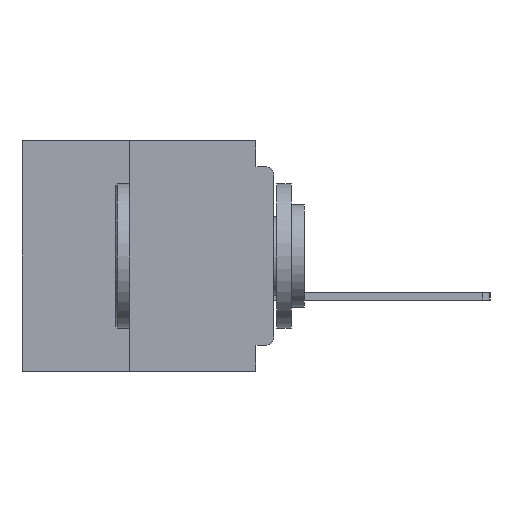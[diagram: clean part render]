
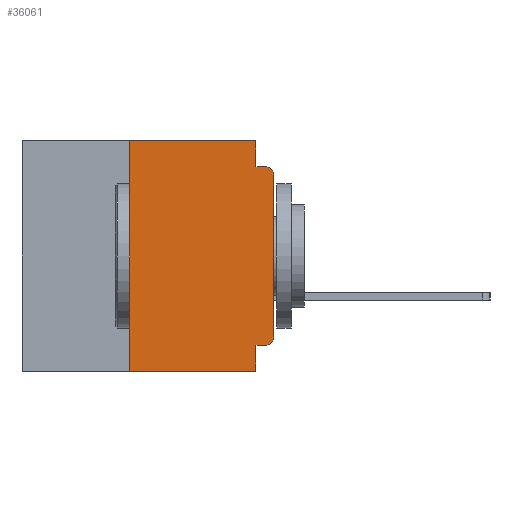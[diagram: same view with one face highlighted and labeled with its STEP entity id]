
A CAD part, left-side view. The second image highlights one B-rep face of the part: STEP entity #36061.
In plain terms, the highlighted planar face has unit normal (-1, 0, 0).
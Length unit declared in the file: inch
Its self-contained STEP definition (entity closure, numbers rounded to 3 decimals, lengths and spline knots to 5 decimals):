
#31 = DIRECTION ( 'NONE',  ( 0., -1., 0. ) ) ;
#459 = ORIENTED_EDGE ( 'NONE', *, *, #33806, .T. ) ;
#517 = DIRECTION ( 'NONE',  ( 0., 0., -1. ) ) ;
#1247 = DIRECTION ( 'NONE',  ( 0., -1., 0. ) ) ;
#2283 = LINE ( 'NONE', #17625, #20515 ) ;
#2712 = VERTEX_POINT ( 'NONE', #13226 ) ;
#4377 = CARTESIAN_POINT ( 'NONE',  ( 0., 0.031, -0.045 ) ) ;
#5106 = VERTEX_POINT ( 'NONE', #21611 ) ;
#5412 = ORIENTED_EDGE ( 'NONE', *, *, #19987, .T. ) ;
#6011 = AXIS2_PLACEMENT_3D ( 'NONE', #10459, #39322, #14601 ) ;
#7656 = CARTESIAN_POINT ( 'NONE',  ( 0., 0.031, 0. ) ) ;
#8273 = LINE ( 'NONE', #52745, #50850 ) ;
#10038 = DIRECTION ( 'NONE',  ( -1., 0., 0. ) ) ;
#10459 = CARTESIAN_POINT ( 'NONE',  ( 0., 0.015, -0.34 ) ) ;
#11101 = VERTEX_POINT ( 'NONE', #41931 ) ;
#11694 = DIRECTION ( 'NONE',  ( 0., 1., 0. ) ) ;
#13226 = CARTESIAN_POINT ( 'NONE',  ( 0., 0., -0.06 ) ) ;
#13695 = CARTESIAN_POINT ( 'NONE',  ( 0., 0.437, 0. ) ) ;
#14601 = DIRECTION ( 'NONE',  ( 0., 0., -1. ) ) ;
#14728 = LINE ( 'NONE', #50128, #35390 ) ;
#15181 = VERTEX_POINT ( 'NONE', #52585 ) ;
#15403 = VERTEX_POINT ( 'NONE', #4377 ) ;
#15664 = DIRECTION ( 'NONE',  ( 0., -1., 0. ) ) ;
#15763 = CIRCLE ( 'NONE', #19614, 0.015 ) ;
#16553 = CARTESIAN_POINT ( 'NONE',  ( 0., 0.437, 0. ) ) ;
#16823 = EDGE_LOOP ( 'NONE', ( #44016, #459, #50328, #39913, #51917, #40638, #39721, #34998, #29249, #5412 ) ) ;
#17018 = CARTESIAN_POINT ( 'NONE',  ( 0., 0.015, -0.045 ) ) ;
#17625 = CARTESIAN_POINT ( 'NONE',  ( 0., 0.25, -0.4 ) ) ;
#18974 = EDGE_CURVE ( 'NONE', #15403, #24343, #45887, .T. ) ;
#19614 = AXIS2_PLACEMENT_3D ( 'NONE', #34772, #10038, #38875 ) ;
#19987 = EDGE_CURVE ( 'NONE', #5106, #11101, #48443, .T. ) ;
#20515 = VECTOR ( 'NONE', #21734, 39.37008 ) ;
#20682 = DIRECTION ( 'NONE',  ( 0., 0., -1. ) ) ;
#21370 = CARTESIAN_POINT ( 'NONE',  ( 0., 0., 0. ) ) ;
#21611 = CARTESIAN_POINT ( 'NONE',  ( 0., 0.015, -0.355 ) ) ;
#21734 = DIRECTION ( 'NONE',  ( 0., 0., 1. ) ) ;
#22354 = EDGE_CURVE ( 'NONE', #48712, #46539, #46209, .T. ) ;
#22435 = AXIS2_PLACEMENT_3D ( 'NONE', #16553, #45345, #20682 ) ;
#22874 = VECTOR ( 'NONE', #15664, 39.37008 ) ;
#24320 = VECTOR ( 'NONE', #11694, 39.37008 ) ;
#24343 = VERTEX_POINT ( 'NONE', #17018 ) ;
#24941 = CARTESIAN_POINT ( 'NONE',  ( 0., 0., -0.045 ) ) ;
#24942 = CARTESIAN_POINT ( 'NONE',  ( 0., 0.25, -0.4 ) ) ;
#25096 = LINE ( 'NONE', #21370, #34847 ) ;
#25546 = VERTEX_POINT ( 'NONE', #24942 ) ;
#27867 = VECTOR ( 'NONE', #31, 39.37008 ) ;
#29249 = ORIENTED_EDGE ( 'NONE', *, *, #50360, .F. ) ;
#30649 = EDGE_CURVE ( 'NONE', #15181, #52900, #8273, .T. ) ;
#33409 = EDGE_CURVE ( 'NONE', #25546, #52900, #33882, .T. ) ;
#33686 = CARTESIAN_POINT ( 'NONE',  ( 0., 0.25, 0. ) ) ;
#33806 = EDGE_CURVE ( 'NONE', #2712, #24343, #15763, .T. ) ;
#33882 = LINE ( 'NONE', #36231, #22874 ) ;
#34772 = CARTESIAN_POINT ( 'NONE',  ( 0., 0.015, -0.06 ) ) ;
#34847 = VECTOR ( 'NONE', #46019, 39.37008 ) ;
#34998 = ORIENTED_EDGE ( 'NONE', *, *, #30649, .F. ) ;
#35305 = VECTOR ( 'NONE', #1247, 39.37008 ) ;
#35390 = VECTOR ( 'NONE', #517, 39.37008 ) ;
#36061 = ADVANCED_FACE ( 'NONE', ( #43195 ), #37090, .F. ) ;
#36231 = CARTESIAN_POINT ( 'NONE',  ( 0., 0.437, -0.4 ) ) ;
#36389 = DIRECTION ( 'NONE',  ( 0., 0., -1. ) ) ;
#37090 = PLANE ( 'NONE',  #22435 ) ;
#37526 = CARTESIAN_POINT ( 'NONE',  ( 0., 0.031, -0.4 ) ) ;
#38875 = DIRECTION ( 'NONE',  ( 0., 0., -1. ) ) ;
#39322 = DIRECTION ( 'NONE',  ( -1., 0., 0. ) ) ;
#39721 = ORIENTED_EDGE ( 'NONE', *, *, #33409, .T. ) ;
#39913 = ORIENTED_EDGE ( 'NONE', *, *, #49967, .F. ) ;
#40638 = ORIENTED_EDGE ( 'NONE', *, *, #44411, .F. ) ;
#41931 = CARTESIAN_POINT ( 'NONE',  ( 0., 0., -0.34 ) ) ;
#43195 = FACE_OUTER_BOUND ( 'NONE', #16823, .T. ) ;
#44016 = ORIENTED_EDGE ( 'NONE', *, *, #49343, .T. ) ;
#44411 = EDGE_CURVE ( 'NONE', #25546, #48712, #2283, .T. ) ;
#45345 = DIRECTION ( 'NONE',  ( 1., 0., 0. ) ) ;
#45887 = LINE ( 'NONE', #24941, #27867 ) ;
#46019 = DIRECTION ( 'NONE',  ( 0., 0., 1. ) ) ;
#46209 = LINE ( 'NONE', #13695, #35305 ) ;
#46539 = VERTEX_POINT ( 'NONE', #7656 ) ;
#47573 = LINE ( 'NONE', #52794, #24320 ) ;
#48443 = CIRCLE ( 'NONE', #6011, 0.015 ) ;
#48712 = VERTEX_POINT ( 'NONE', #33686 ) ;
#49343 = EDGE_CURVE ( 'NONE', #11101, #2712, #25096, .T. ) ;
#49967 = EDGE_CURVE ( 'NONE', #46539, #15403, #14728, .T. ) ;
#50128 = CARTESIAN_POINT ( 'NONE',  ( 0., 0.031, 0. ) ) ;
#50328 = ORIENTED_EDGE ( 'NONE', *, *, #18974, .F. ) ;
#50360 = EDGE_CURVE ( 'NONE', #5106, #15181, #47573, .T. ) ;
#50850 = VECTOR ( 'NONE', #36389, 39.37008 ) ;
#51917 = ORIENTED_EDGE ( 'NONE', *, *, #22354, .F. ) ;
#52585 = CARTESIAN_POINT ( 'NONE',  ( 0., 0.031, -0.355 ) ) ;
#52745 = CARTESIAN_POINT ( 'NONE',  ( 0., 0.031, -0.4 ) ) ;
#52794 = CARTESIAN_POINT ( 'NONE',  ( 0., 0., -0.355 ) ) ;
#52900 = VERTEX_POINT ( 'NONE', #37526 ) ;
